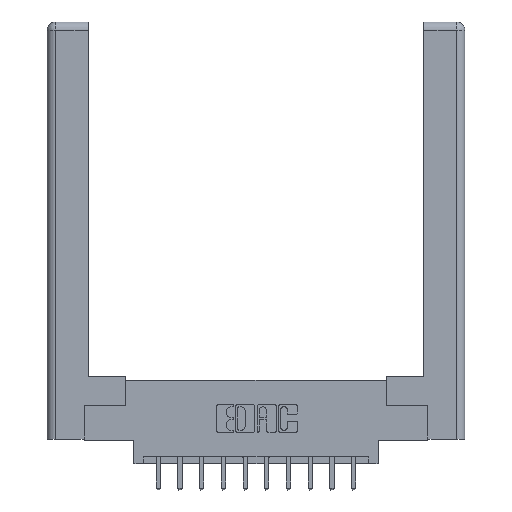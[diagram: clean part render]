
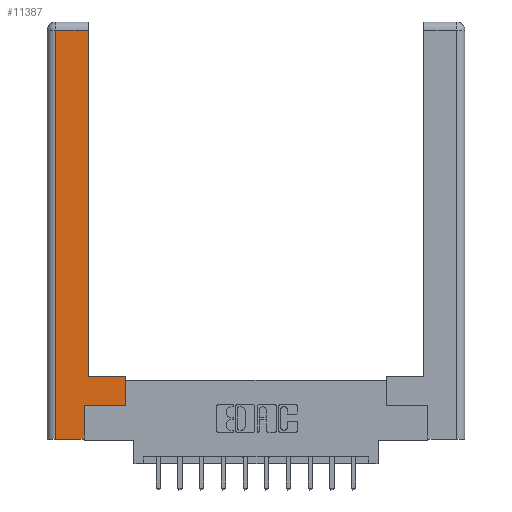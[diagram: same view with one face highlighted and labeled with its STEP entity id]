
A CAD part, top view. The second image highlights one B-rep face of the part: STEP entity #11387.
In plain terms, the highlighted planar face has unit normal (0, 0, 1).
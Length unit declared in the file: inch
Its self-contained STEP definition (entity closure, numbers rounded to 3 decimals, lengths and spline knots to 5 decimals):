
#252 = ORIENTED_EDGE ( 'NONE', *, *, #3705, .T. ) ;
#681 = CARTESIAN_POINT ( 'NONE',  ( 0.265, 0.245, 0. ) ) ;
#874 = DIRECTION ( 'NONE',  ( -1., 0., 0. ) ) ;
#1072 = ORIENTED_EDGE ( 'NONE', *, *, #8392, .T. ) ;
#1078 = FACE_OUTER_BOUND ( 'NONE', #13661, .T. ) ;
#1387 = DIRECTION ( 'NONE',  ( -1., 0., 0. ) ) ;
#1768 = VECTOR ( 'NONE', #2633, 39.37008 ) ;
#2320 = ORIENTED_EDGE ( 'NONE', *, *, #4885, .T. ) ;
#2632 = PLANE ( 'NONE',  #10860 ) ;
#2633 = DIRECTION ( 'NONE',  ( 0., -1., 0. ) ) ;
#2640 = CARTESIAN_POINT ( 'NONE',  ( 0.295, 2.94, 0. ) ) ;
#3165 = DIRECTION ( 'NONE',  ( 0., 1., 0. ) ) ;
#3415 = EDGE_CURVE ( 'NONE', #7913, #6998, #9738, .T. ) ;
#3499 = CARTESIAN_POINT ( 'NONE',  ( 0.0615, 2.94, 0. ) ) ;
#3529 = ORIENTED_EDGE ( 'NONE', *, *, #9080, .T. ) ;
#3705 = EDGE_CURVE ( 'NONE', #10076, #6106, #10246, .T. ) ;
#3795 = DIRECTION ( 'NONE',  ( -1., 0., 0. ) ) ;
#4070 = LINE ( 'NONE', #5849, #12157 ) ;
#4298 = EDGE_CURVE ( 'NONE', #6998, #11923, #6616, .T. ) ;
#4407 = DIRECTION ( 'NONE',  ( 0., 1., 0. ) ) ;
#4597 = CARTESIAN_POINT ( 'NONE',  ( 0.265, 0.245, 0. ) ) ;
#4721 = VERTEX_POINT ( 'NONE', #6815 ) ;
#4803 = LINE ( 'NONE', #14064, #1768 ) ;
#4885 = EDGE_CURVE ( 'NONE', #6198, #4721, #12727, .T. ) ;
#4887 = CARTESIAN_POINT ( 'NONE',  ( 0.565, 0.45, 0. ) ) ;
#4983 = DIRECTION ( 'NONE',  ( 0., 0., -1. ) ) ;
#5639 = ORIENTED_EDGE ( 'NONE', *, *, #6909, .T. ) ;
#5849 = CARTESIAN_POINT ( 'NONE',  ( 0.565, 0.245, 0. ) ) ;
#5945 = DIRECTION ( 'NONE',  ( 1., 0., 0. ) ) ;
#6106 = VERTEX_POINT ( 'NONE', #3499 ) ;
#6198 = VERTEX_POINT ( 'NONE', #12706 ) ;
#6473 = VERTEX_POINT ( 'NONE', #681 ) ;
#6602 = VECTOR ( 'NONE', #13092, 39.37008 ) ;
#6616 = LINE ( 'NONE', #12919, #11472 ) ;
#6815 = CARTESIAN_POINT ( 'NONE',  ( 0.265, 0., 0. ) ) ;
#6909 = EDGE_CURVE ( 'NONE', #6473, #7913, #4070, .T. ) ;
#6998 = VERTEX_POINT ( 'NONE', #4887 ) ;
#7913 = VERTEX_POINT ( 'NONE', #10278 ) ;
#8140 = CARTESIAN_POINT ( 'NONE',  ( 0.265, 0., 0. ) ) ;
#8392 = EDGE_CURVE ( 'NONE', #11923, #10076, #9683, .T. ) ;
#8647 = CARTESIAN_POINT ( 'NONE',  ( 0.0615, 2.94, 0. ) ) ;
#9080 = EDGE_CURVE ( 'NONE', #4721, #6473, #12616, .T. ) ;
#9157 = ORIENTED_EDGE ( 'NONE', *, *, #4298, .T. ) ;
#9357 = VECTOR ( 'NONE', #3165, 39.37008 ) ;
#9683 = LINE ( 'NONE', #10144, #13962 ) ;
#9738 = LINE ( 'NONE', #13475, #9357 ) ;
#10076 = VERTEX_POINT ( 'NONE', #2640 ) ;
#10144 = CARTESIAN_POINT ( 'NONE',  ( 0.295, 3., 0. ) ) ;
#10246 = LINE ( 'NONE', #8647, #13658 ) ;
#10278 = CARTESIAN_POINT ( 'NONE',  ( 0.565, 0.245, 0. ) ) ;
#10656 = CARTESIAN_POINT ( 'NONE',  ( 0., 0., 0. ) ) ;
#10860 = AXIS2_PLACEMENT_3D ( 'NONE', #10656, #4983, #3795 ) ;
#11338 = ORIENTED_EDGE ( 'NONE', *, *, #3415, .T. ) ;
#11387 = ADVANCED_FACE ( 'NONE', ( #1078 ), #2632, .F. ) ;
#11472 = VECTOR ( 'NONE', #1387, 39.37008 ) ;
#11923 = VERTEX_POINT ( 'NONE', #14669 ) ;
#12099 = ORIENTED_EDGE ( 'NONE', *, *, #13086, .T. ) ;
#12157 = VECTOR ( 'NONE', #5945, 39.37008 ) ;
#12616 = LINE ( 'NONE', #4597, #13163 ) ;
#12706 = CARTESIAN_POINT ( 'NONE',  ( 0.0615, 0., 0. ) ) ;
#12727 = LINE ( 'NONE', #8140, #6602 ) ;
#12919 = CARTESIAN_POINT ( 'NONE',  ( 0.295, 0.45, 0. ) ) ;
#13086 = EDGE_CURVE ( 'NONE', #6106, #6198, #4803, .T. ) ;
#13092 = DIRECTION ( 'NONE',  ( 1., 0., 0. ) ) ;
#13163 = VECTOR ( 'NONE', #13788, 39.37008 ) ;
#13475 = CARTESIAN_POINT ( 'NONE',  ( 0.565, 0.45, 0. ) ) ;
#13658 = VECTOR ( 'NONE', #874, 39.37008 ) ;
#13661 = EDGE_LOOP ( 'NONE', ( #1072, #252, #12099, #2320, #3529, #5639, #11338, #9157 ) ) ;
#13788 = DIRECTION ( 'NONE',  ( 0., 1., 0. ) ) ;
#13962 = VECTOR ( 'NONE', #4407, 39.37008 ) ;
#14064 = CARTESIAN_POINT ( 'NONE',  ( 0.0615, 0., 0. ) ) ;
#14669 = CARTESIAN_POINT ( 'NONE',  ( 0.295, 0.45, 0. ) ) ;
